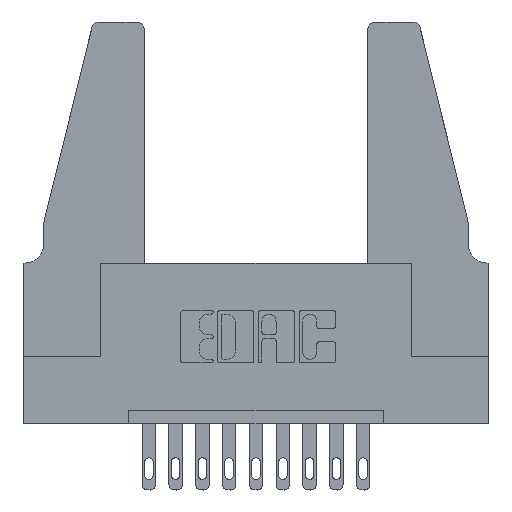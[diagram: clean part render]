
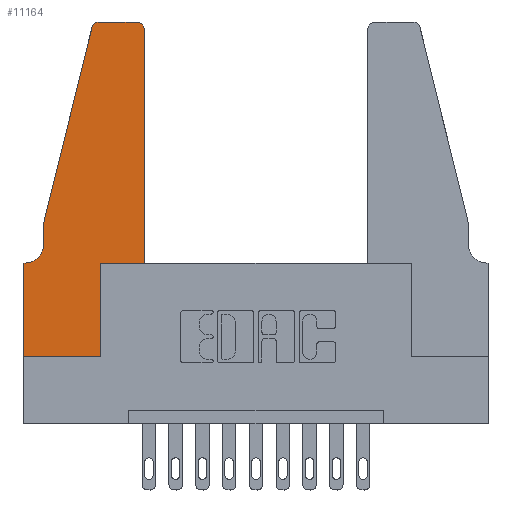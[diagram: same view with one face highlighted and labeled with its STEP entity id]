
A CAD part, top view. The second image highlights one B-rep face of the part: STEP entity #11164.
In plain terms, the highlighted planar face has unit normal (0, 0, 1).
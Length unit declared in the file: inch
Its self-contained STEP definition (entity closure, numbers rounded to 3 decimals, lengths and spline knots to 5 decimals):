
#31 = VECTOR ( 'NONE', #8251, 39.37008 ) ;
#106 = CARTESIAN_POINT ( 'NONE',  ( 0.0755, 0.42, 0.37 ) ) ;
#128 = EDGE_CURVE ( 'NONE', #4475, #11247, #9812, .T. ) ;
#357 = DIRECTION ( 'NONE',  ( 0., 1., 0. ) ) ;
#362 = CIRCLE ( 'NONE', #8485, 0.03 ) ;
#370 = VERTEX_POINT ( 'NONE', #1512 ) ;
#486 = VERTEX_POINT ( 'NONE', #10391 ) ;
#757 = CIRCLE ( 'NONE', #5488, 0.07 ) ;
#995 = ORIENTED_EDGE ( 'NONE', *, *, #5440, .T. ) ;
#1055 = ORIENTED_EDGE ( 'NONE', *, *, #3568, .T. ) ;
#1481 = VERTEX_POINT ( 'NONE', #3767 ) ;
#1512 = CARTESIAN_POINT ( 'NONE',  ( 0.0055, 0.35, 0.37 ) ) ;
#1603 = ORIENTED_EDGE ( 'NONE', *, *, #128, .T. ) ;
#1646 = VECTOR ( 'NONE', #12664, 39.37008 ) ;
#1773 = DIRECTION ( 'NONE',  ( 0., 0., -1. ) ) ;
#1989 = LINE ( 'NONE', #6828, #7127 ) ;
#2071 = CARTESIAN_POINT ( 'NONE',  ( 0.4205, 1.22, 0.37 ) ) ;
#2118 = LINE ( 'NONE', #7375, #31 ) ;
#2245 = VERTEX_POINT ( 'NONE', #8305 ) ;
#2283 = VECTOR ( 'NONE', #7481, 39.37008 ) ;
#2450 = EDGE_LOOP ( 'NONE', ( #995, #4308, #2496, #1603, #10551, #11580, #1055, #5097, #10102, #9061, #13100, #6906 ) ) ;
#2496 = ORIENTED_EDGE ( 'NONE', *, *, #9297, .T. ) ;
#2785 = LINE ( 'NONE', #4342, #8417 ) ;
#2934 = CARTESIAN_POINT ( 'NONE',  ( 0.0755, 0.35, 0.37 ) ) ;
#2954 = EDGE_CURVE ( 'NONE', #2245, #10309, #8585, .T. ) ;
#3090 = DIRECTION ( 'NONE',  ( 1., 0., 0. ) ) ;
#3106 = AXIS2_PLACEMENT_3D ( 'NONE', #11210, #5118, #12250 ) ;
#3116 = DIRECTION ( 'NONE',  ( 1., 0., 0. ) ) ;
#3432 = VERTEX_POINT ( 'NONE', #7992 ) ;
#3440 = LINE ( 'NONE', #6399, #1646 ) ;
#3510 = DIRECTION ( 'NONE',  ( -0.239, -0.971, 0. ) ) ;
#3568 = EDGE_CURVE ( 'NONE', #5788, #3432, #3440, .T. ) ;
#3574 = DIRECTION ( 'NONE',  ( 0., 1., 0. ) ) ;
#3767 = CARTESIAN_POINT ( 'NONE',  ( 0.25487, 1.22718, 0.37 ) ) ;
#4238 = EDGE_CURVE ( 'NONE', #10309, #13197, #2785, .T. ) ;
#4308 = ORIENTED_EDGE ( 'NONE', *, *, #6576, .T. ) ;
#4342 = CARTESIAN_POINT ( 'NONE',  ( 0.4505, 0.35, 0.37 ) ) ;
#4475 = VERTEX_POINT ( 'NONE', #12028 ) ;
#4572 = VERTEX_POINT ( 'NONE', #11571 ) ;
#4587 = CARTESIAN_POINT ( 'NONE',  ( 0.0755, 0.5, 0.37 ) ) ;
#4620 = DIRECTION ( 'NONE',  ( 0., -1., 0. ) ) ;
#4842 = CARTESIAN_POINT ( 'NONE',  ( 0., 0., 0.37 ) ) ;
#5092 = EDGE_CURVE ( 'NONE', #370, #5788, #12114, .T. ) ;
#5097 = ORIENTED_EDGE ( 'NONE', *, *, #6713, .T. ) ;
#5118 = DIRECTION ( 'NONE',  ( 0., 0., 1. ) ) ;
#5440 = EDGE_CURVE ( 'NONE', #486, #5981, #2118, .T. ) ;
#5488 = AXIS2_PLACEMENT_3D ( 'NONE', #5881, #1773, #10063 ) ;
#5709 = CARTESIAN_POINT ( 'NONE',  ( 0.284, 1.22, 0.37 ) ) ;
#5788 = VERTEX_POINT ( 'NONE', #10064 ) ;
#5881 = CARTESIAN_POINT ( 'NONE',  ( 0.0055, 0.42, 0.37 ) ) ;
#5981 = VERTEX_POINT ( 'NONE', #12039 ) ;
#6399 = CARTESIAN_POINT ( 'NONE',  ( 0., 0., 0.37 ) ) ;
#6576 = EDGE_CURVE ( 'NONE', #5981, #1481, #362, .T. ) ;
#6661 = FACE_OUTER_BOUND ( 'NONE', #2450, .T. ) ;
#6713 = EDGE_CURVE ( 'NONE', #3432, #4572, #11157, .T. ) ;
#6739 = VECTOR ( 'NONE', #4620, 39.37008 ) ;
#6828 = CARTESIAN_POINT ( 'NONE',  ( 0.2865, 0.35, 0.37 ) ) ;
#6906 = ORIENTED_EDGE ( 'NONE', *, *, #12645, .T. ) ;
#7127 = VECTOR ( 'NONE', #3574, 39.37008 ) ;
#7161 = PLANE ( 'NONE',  #3106 ) ;
#7375 = CARTESIAN_POINT ( 'NONE',  ( 0.2605, 1.25, 0.37 ) ) ;
#7481 = DIRECTION ( 'NONE',  ( -1., 0., 0. ) ) ;
#7620 = VECTOR ( 'NONE', #3090, 39.37008 ) ;
#7664 = CARTESIAN_POINT ( 'NONE',  ( 0.4505, 0.35, 0.37 ) ) ;
#7964 = DIRECTION ( 'NONE',  ( 1., 0., 0. ) ) ;
#7992 = CARTESIAN_POINT ( 'NONE',  ( 0., 0., 0.37 ) ) ;
#8251 = DIRECTION ( 'NONE',  ( -1., 0., 0. ) ) ;
#8305 = CARTESIAN_POINT ( 'NONE',  ( 0.2865, 0.35, 0.37 ) ) ;
#8417 = VECTOR ( 'NONE', #357, 39.37008 ) ;
#8485 = AXIS2_PLACEMENT_3D ( 'NONE', #5709, #12053, #12012 ) ;
#8585 = LINE ( 'NONE', #11353, #7620 ) ;
#8907 = CARTESIAN_POINT ( 'NONE',  ( 0.0755, 0.5, 0.37 ) ) ;
#9061 = ORIENTED_EDGE ( 'NONE', *, *, #2954, .T. ) ;
#9173 = CARTESIAN_POINT ( 'NONE',  ( 0.4505, 1.22, 0.37 ) ) ;
#9297 = EDGE_CURVE ( 'NONE', #1481, #4475, #10750, .T. ) ;
#9420 = CIRCLE ( 'NONE', #12587, 0.03 ) ;
#9751 = EDGE_CURVE ( 'NONE', #11247, #370, #757, .T. ) ;
#9812 = LINE ( 'NONE', #8907, #6739 ) ;
#10063 = DIRECTION ( 'NONE',  ( -1., 0., 0. ) ) ;
#10064 = CARTESIAN_POINT ( 'NONE',  ( 0., 0.35, 0.37 ) ) ;
#10102 = ORIENTED_EDGE ( 'NONE', *, *, #12339, .T. ) ;
#10309 = VERTEX_POINT ( 'NONE', #7664 ) ;
#10344 = DIRECTION ( 'NONE',  ( 0., 0., 1. ) ) ;
#10391 = CARTESIAN_POINT ( 'NONE',  ( 0.4205, 1.25, 0.37 ) ) ;
#10447 = VECTOR ( 'NONE', #3510, 39.37008 ) ;
#10551 = ORIENTED_EDGE ( 'NONE', *, *, #9751, .T. ) ;
#10750 = LINE ( 'NONE', #4587, #10447 ) ;
#11157 = LINE ( 'NONE', #4842, #13085 ) ;
#11164 = ADVANCED_FACE ( 'NONE', ( #6661 ), #7161, .T. ) ;
#11210 = CARTESIAN_POINT ( 'NONE',  ( 0., 0.35, 0.37 ) ) ;
#11247 = VERTEX_POINT ( 'NONE', #106 ) ;
#11353 = CARTESIAN_POINT ( 'NONE',  ( 0.4505, 0.35, 0.37 ) ) ;
#11571 = CARTESIAN_POINT ( 'NONE',  ( 0.2865, 0., 0.37 ) ) ;
#11580 = ORIENTED_EDGE ( 'NONE', *, *, #5092, .T. ) ;
#12012 = DIRECTION ( 'NONE',  ( 1., 0., 0. ) ) ;
#12028 = CARTESIAN_POINT ( 'NONE',  ( 0.0755, 0.5, 0.37 ) ) ;
#12039 = CARTESIAN_POINT ( 'NONE',  ( 0.284, 1.25, 0.37 ) ) ;
#12053 = DIRECTION ( 'NONE',  ( 0., 0., 1. ) ) ;
#12114 = LINE ( 'NONE', #2934, #2283 ) ;
#12250 = DIRECTION ( 'NONE',  ( 1., 0., 0. ) ) ;
#12339 = EDGE_CURVE ( 'NONE', #4572, #2245, #1989, .T. ) ;
#12587 = AXIS2_PLACEMENT_3D ( 'NONE', #2071, #10344, #3116 ) ;
#12645 = EDGE_CURVE ( 'NONE', #13197, #486, #9420, .T. ) ;
#12664 = DIRECTION ( 'NONE',  ( 0., -1., 0. ) ) ;
#13085 = VECTOR ( 'NONE', #7964, 39.37008 ) ;
#13100 = ORIENTED_EDGE ( 'NONE', *, *, #4238, .T. ) ;
#13197 = VERTEX_POINT ( 'NONE', #9173 ) ;
